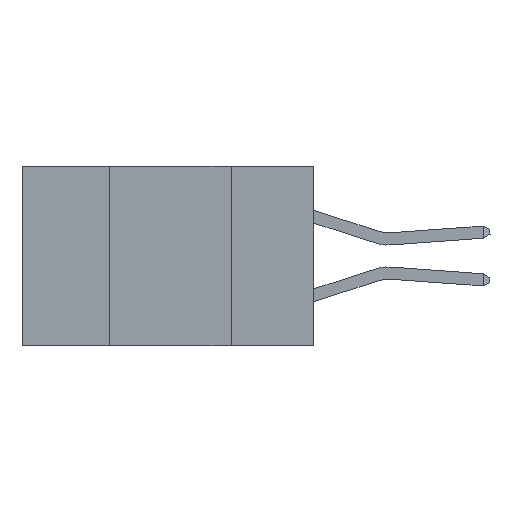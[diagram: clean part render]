
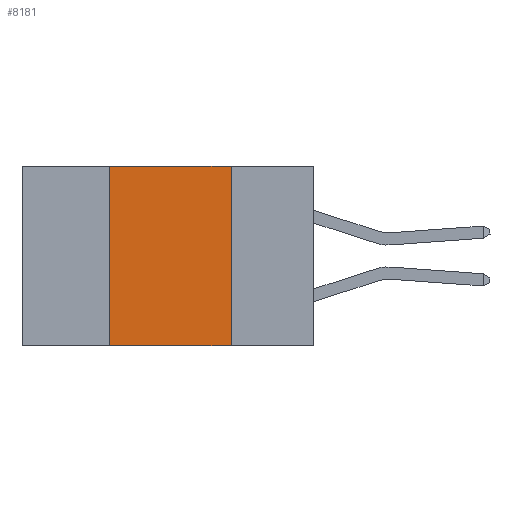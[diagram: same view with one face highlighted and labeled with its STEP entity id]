
A CAD part, left-side view. The second image highlights one B-rep face of the part: STEP entity #8181.
In plain terms, the highlighted planar face has unit normal (-1, 0, 0).
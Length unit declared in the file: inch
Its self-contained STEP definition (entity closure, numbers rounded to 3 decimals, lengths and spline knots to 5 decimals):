
#722 = LINE ( 'NONE', #9813, #7565 ) ;
#829 = EDGE_CURVE ( 'NONE', #9287, #7363, #1466, .T. ) ;
#1466 = LINE ( 'NONE', #8874, #5393 ) ;
#1509 = ORIENTED_EDGE ( 'NONE', *, *, #829, .F. ) ;
#1584 = DIRECTION ( 'NONE',  ( 0., 0., 1. ) ) ;
#3126 = VERTEX_POINT ( 'NONE', #7855 ) ;
#3208 = EDGE_CURVE ( 'NONE', #3126, #7363, #722, .T. ) ;
#3353 = FACE_OUTER_BOUND ( 'NONE', #4412, .T. ) ;
#4228 = ORIENTED_EDGE ( 'NONE', *, *, #3208, .T. ) ;
#4378 = CARTESIAN_POINT ( 'NONE',  ( 0., 0.6, 0. ) ) ;
#4412 = EDGE_LOOP ( 'NONE', ( #1509, #5543, #8124, #4228 ) ) ;
#5170 = CARTESIAN_POINT ( 'NONE',  ( 0., 0.17, -0.37 ) ) ;
#5279 = CARTESIAN_POINT ( 'NONE',  ( 0., 0.6, 0. ) ) ;
#5280 = PLANE ( 'NONE',  #9363 ) ;
#5393 = VECTOR ( 'NONE', #10836, 39.37008 ) ;
#5543 = ORIENTED_EDGE ( 'NONE', *, *, #10626, .F. ) ;
#6496 = VECTOR ( 'NONE', #1584, 39.37008 ) ;
#7105 = DIRECTION ( 'NONE',  ( 0., 0., -1. ) ) ;
#7363 = VERTEX_POINT ( 'NONE', #5170 ) ;
#7565 = VECTOR ( 'NONE', #9054, 39.37008 ) ;
#7855 = CARTESIAN_POINT ( 'NONE',  ( 0., 0.42, -0.37 ) ) ;
#8124 = ORIENTED_EDGE ( 'NONE', *, *, #11172, .F. ) ;
#8181 = ADVANCED_FACE ( 'NONE', ( #3353 ), #5280, .F. ) ;
#8334 = LINE ( 'NONE', #11300, #6496 ) ;
#8644 = VECTOR ( 'NONE', #11590, 39.37008 ) ;
#8658 = CARTESIAN_POINT ( 'NONE',  ( 0., 0.42, 0. ) ) ;
#8802 = VERTEX_POINT ( 'NONE', #8658 ) ;
#8874 = CARTESIAN_POINT ( 'NONE',  ( 0., 0.17, 0. ) ) ;
#9054 = DIRECTION ( 'NONE',  ( 0., -1., 0. ) ) ;
#9287 = VERTEX_POINT ( 'NONE', #10202 ) ;
#9363 = AXIS2_PLACEMENT_3D ( 'NONE', #4378, #10610, #7105 ) ;
#9371 = LINE ( 'NONE', #5279, #8644 ) ;
#9813 = CARTESIAN_POINT ( 'NONE',  ( 0., 0.6, -0.37 ) ) ;
#10202 = CARTESIAN_POINT ( 'NONE',  ( 0., 0.17, 0. ) ) ;
#10610 = DIRECTION ( 'NONE',  ( 1., 0., 0. ) ) ;
#10626 = EDGE_CURVE ( 'NONE', #8802, #9287, #9371, .T. ) ;
#10836 = DIRECTION ( 'NONE',  ( 0., 0., -1. ) ) ;
#11172 = EDGE_CURVE ( 'NONE', #3126, #8802, #8334, .T. ) ;
#11300 = CARTESIAN_POINT ( 'NONE',  ( 0., 0.42, 0. ) ) ;
#11590 = DIRECTION ( 'NONE',  ( 0., -1., 0. ) ) ;
